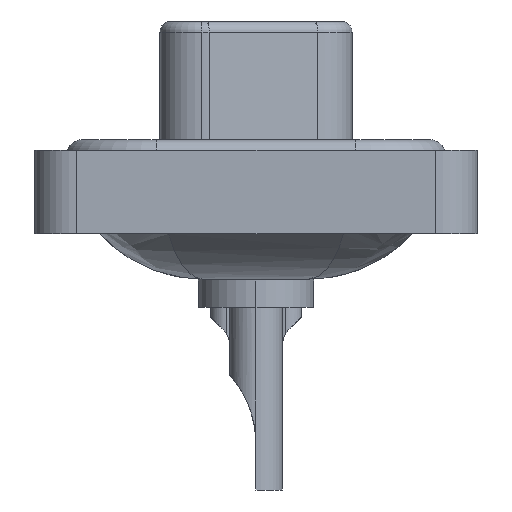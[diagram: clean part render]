
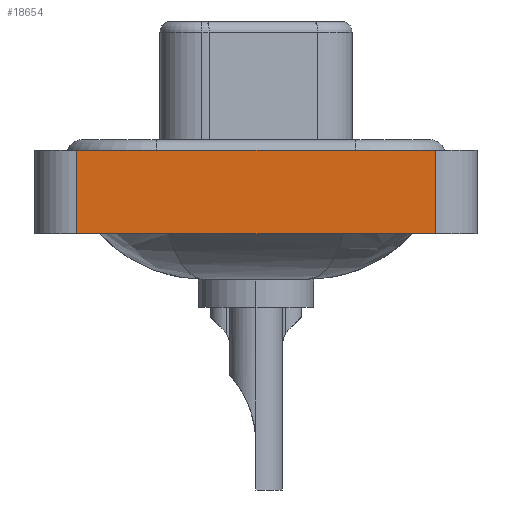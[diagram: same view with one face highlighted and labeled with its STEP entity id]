
A CAD part, left-side view. The second image highlights one B-rep face of the part: STEP entity #18654.
In plain terms, the highlighted planar face has unit normal (-1, 0, 0).
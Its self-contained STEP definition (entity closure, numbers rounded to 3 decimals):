
#151 = VECTOR ( 'NONE', #19292, 1000. ) ;
#1184 = ORIENTED_EDGE ( 'NONE', *, *, #10330, .T. ) ;
#2317 = PLANE ( 'NONE',  #13535 ) ;
#2652 = LINE ( 'NONE', #17868, #5299 ) ;
#2691 = CARTESIAN_POINT ( 'NONE',  ( -7.35, -8.55, 0.4 ) ) ;
#3109 = EDGE_CURVE ( 'NONE', #12862, #8109, #19814, .T. ) ;
#3238 = VECTOR ( 'NONE', #12856, 1000. ) ;
#3414 = CARTESIAN_POINT ( 'NONE',  ( -7.35, -8.55, -3.6 ) ) ;
#3955 = DIRECTION ( 'NONE',  ( 0., 0., 1. ) ) ;
#4419 = EDGE_CURVE ( 'NONE', #8109, #8531, #9214, .T. ) ;
#4583 = DIRECTION ( 'NONE',  ( 0., 0., 1. ) ) ;
#4665 = CARTESIAN_POINT ( 'NONE',  ( -7.35, -8.55, -3.6 ) ) ;
#4902 = ORIENTED_EDGE ( 'NONE', *, *, #8094, .T. ) ;
#5299 = VECTOR ( 'NONE', #6000, 1000. ) ;
#6000 = DIRECTION ( 'NONE',  ( 0., 0., 1. ) ) ;
#8094 = EDGE_CURVE ( 'NONE', #12862, #13067, #16088, .T. ) ;
#8109 = VERTEX_POINT ( 'NONE', #19466 ) ;
#8531 = VERTEX_POINT ( 'NONE', #2691 ) ;
#9214 = LINE ( 'NONE', #19194, #151 ) ;
#10330 = EDGE_CURVE ( 'NONE', #13067, #8531, #2652, .T. ) ;
#11582 = CARTESIAN_POINT ( 'NONE',  ( -7.35, 8.55, -3.6 ) ) ;
#12616 = CARTESIAN_POINT ( 'NONE',  ( -7.35, 8.55, -3.6 ) ) ;
#12775 = ORIENTED_EDGE ( 'NONE', *, *, #3109, .F. ) ;
#12856 = DIRECTION ( 'NONE',  ( 0., -1., 0. ) ) ;
#12862 = VERTEX_POINT ( 'NONE', #12616 ) ;
#13067 = VERTEX_POINT ( 'NONE', #3414 ) ;
#13535 = AXIS2_PLACEMENT_3D ( 'NONE', #15794, #17428, #3955 ) ;
#14881 = VECTOR ( 'NONE', #4583, 1000. ) ;
#14973 = ORIENTED_EDGE ( 'NONE', *, *, #4419, .F. ) ;
#15794 = CARTESIAN_POINT ( 'NONE',  ( -7.35, -8.55, -3.6 ) ) ;
#16088 = LINE ( 'NONE', #4665, #3238 ) ;
#17339 = EDGE_LOOP ( 'NONE', ( #1184, #14973, #12775, #4902 ) ) ;
#17428 = DIRECTION ( 'NONE',  ( -1., 0., 0. ) ) ;
#17868 = CARTESIAN_POINT ( 'NONE',  ( -7.35, -8.55, -3.6 ) ) ;
#18654 = ADVANCED_FACE ( 'NONE', ( #18842 ), #2317, .T. ) ;
#18842 = FACE_OUTER_BOUND ( 'NONE', #17339, .T. ) ;
#19194 = CARTESIAN_POINT ( 'NONE',  ( -7.35, -8.55, 0.4 ) ) ;
#19292 = DIRECTION ( 'NONE',  ( 0., -1., 0. ) ) ;
#19466 = CARTESIAN_POINT ( 'NONE',  ( -7.35, 8.55, 0.4 ) ) ;
#19814 = LINE ( 'NONE', #11582, #14881 ) ;
